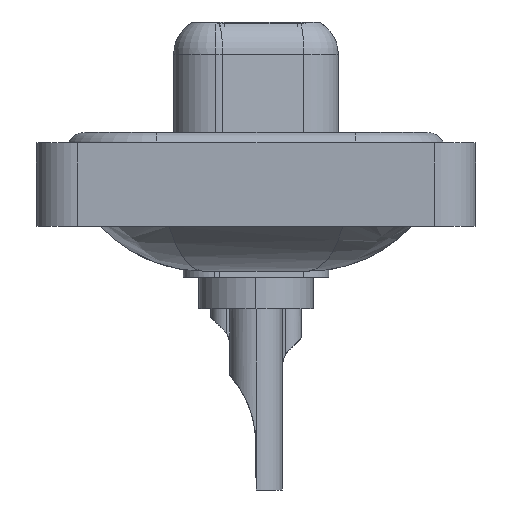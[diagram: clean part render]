
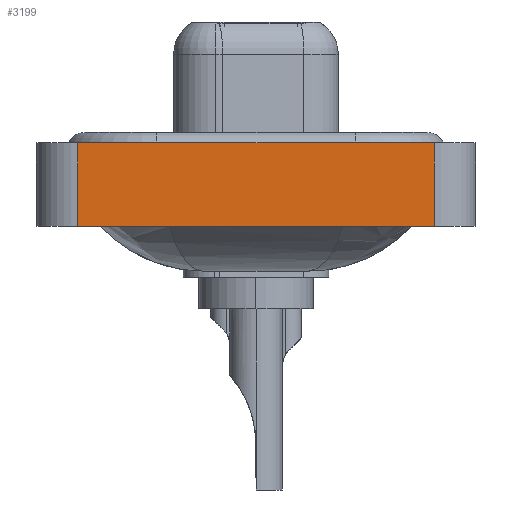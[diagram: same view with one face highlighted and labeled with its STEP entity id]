
A CAD part, left-side view. The second image highlights one B-rep face of the part: STEP entity #3199.
In plain terms, the highlighted planar face has unit normal (-1, 0, 0).
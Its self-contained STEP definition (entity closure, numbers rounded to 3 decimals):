
#866 = LINE ( 'NONE', #9596, #12921 ) ;
#875 = CARTESIAN_POINT ( 'NONE',  ( -7.35, -8.55, 0.4 ) ) ;
#1049 = LINE ( 'NONE', #9685, #21539 ) ;
#1682 = LINE ( 'NONE', #21065, #19900 ) ;
#2446 = CARTESIAN_POINT ( 'NONE',  ( -7.35, -8.55, -3.6 ) ) ;
#3199 = ADVANCED_FACE ( 'NONE', ( #7440 ), #11129, .T. ) ;
#5788 = LINE ( 'NONE', #9023, #8624 ) ;
#5821 = DIRECTION ( 'NONE',  ( -1., 0., 0. ) ) ;
#6625 = ORIENTED_EDGE ( 'NONE', *, *, #21680, .T. ) ;
#7283 = VERTEX_POINT ( 'NONE', #2446 ) ;
#7440 = FACE_OUTER_BOUND ( 'NONE', #21108, .T. ) ;
#8624 = VECTOR ( 'NONE', #16420, 1000. ) ;
#9023 = CARTESIAN_POINT ( 'NONE',  ( -7.35, -8.55, -3.6 ) ) ;
#9596 = CARTESIAN_POINT ( 'NONE',  ( -7.35, -8.55, 0.4 ) ) ;
#9685 = CARTESIAN_POINT ( 'NONE',  ( -7.35, -8.55, -3.6 ) ) ;
#10157 = VERTEX_POINT ( 'NONE', #22174 ) ;
#10235 = ORIENTED_EDGE ( 'NONE', *, *, #21641, .T. ) ;
#10370 = CARTESIAN_POINT ( 'NONE',  ( -7.35, 8.55, -3.6 ) ) ;
#11129 = PLANE ( 'NONE',  #12683 ) ;
#11304 = VERTEX_POINT ( 'NONE', #875 ) ;
#12683 = AXIS2_PLACEMENT_3D ( 'NONE', #20136, #5821, #14717 ) ;
#12921 = VECTOR ( 'NONE', #18629, 1000. ) ;
#13908 = DIRECTION ( 'NONE',  ( 0., 0., 1. ) ) ;
#14717 = DIRECTION ( 'NONE',  ( 0., 0., 1. ) ) ;
#14872 = EDGE_CURVE ( 'NONE', #17910, #10157, #1682, .T. ) ;
#16420 = DIRECTION ( 'NONE',  ( 0., 0., 1. ) ) ;
#16524 = DIRECTION ( 'NONE',  ( 0., -1., 0. ) ) ;
#17910 = VERTEX_POINT ( 'NONE', #10370 ) ;
#18629 = DIRECTION ( 'NONE',  ( 0., -1., 0. ) ) ;
#19900 = VECTOR ( 'NONE', #13908, 1000. ) ;
#20136 = CARTESIAN_POINT ( 'NONE',  ( -7.35, -8.55, -3.6 ) ) ;
#21065 = CARTESIAN_POINT ( 'NONE',  ( -7.35, 8.55, -3.6 ) ) ;
#21108 = EDGE_LOOP ( 'NONE', ( #10235, #22322, #22130, #6625 ) ) ;
#21539 = VECTOR ( 'NONE', #16524, 1000. ) ;
#21641 = EDGE_CURVE ( 'NONE', #7283, #11304, #5788, .T. ) ;
#21680 = EDGE_CURVE ( 'NONE', #17910, #7283, #1049, .T. ) ;
#22130 = ORIENTED_EDGE ( 'NONE', *, *, #14872, .F. ) ;
#22174 = CARTESIAN_POINT ( 'NONE',  ( -7.35, 8.55, 0.4 ) ) ;
#22322 = ORIENTED_EDGE ( 'NONE', *, *, #22567, .F. ) ;
#22567 = EDGE_CURVE ( 'NONE', #10157, #11304, #866, .T. ) ;
